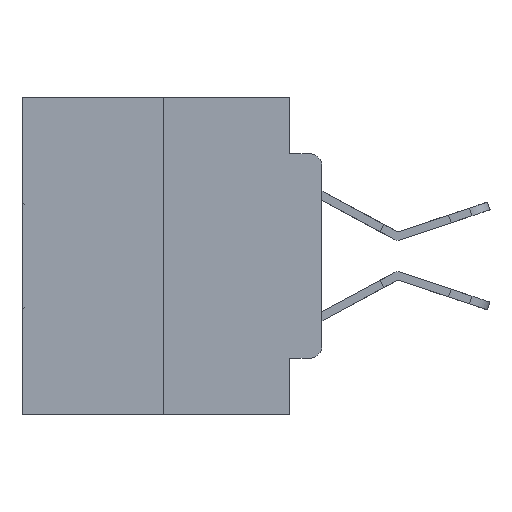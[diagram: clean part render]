
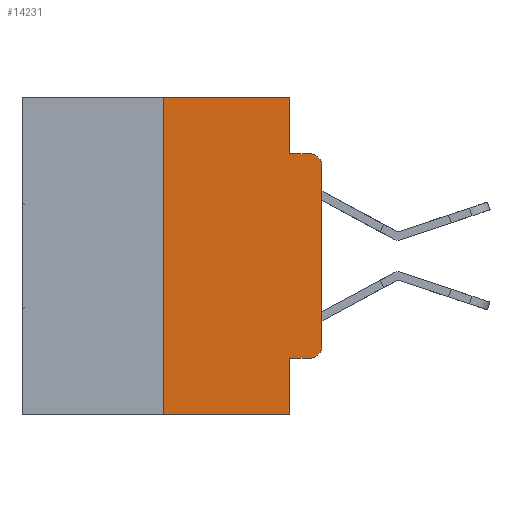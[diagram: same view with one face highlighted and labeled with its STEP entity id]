
A CAD part, left-side view. The second image highlights one B-rep face of the part: STEP entity #14231.
In plain terms, the highlighted planar face has unit normal (-1, 0, 0).
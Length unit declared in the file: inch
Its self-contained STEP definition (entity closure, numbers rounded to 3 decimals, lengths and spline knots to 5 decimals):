
#602 = DIRECTION ( 'NONE',  ( 0., 0., -1. ) ) ;
#644 = CIRCLE ( 'NONE', #16068, 0.02 ) ;
#1045 = ORIENTED_EDGE ( 'NONE', *, *, #2347, .T. ) ;
#1165 = DIRECTION ( 'NONE',  ( 0., -1., 0. ) ) ;
#1322 = LINE ( 'NONE', #6873, #21077 ) ;
#1417 = CARTESIAN_POINT ( 'NONE',  ( 0., 0.051, -0.4115 ) ) ;
#1488 = CARTESIAN_POINT ( 'NONE',  ( 0., 0.051, 0. ) ) ;
#1620 = AXIS2_PLACEMENT_3D ( 'NONE', #18826, #17984, #8869 ) ;
#1840 = ORIENTED_EDGE ( 'NONE', *, *, #3975, .T. ) ;
#2347 = EDGE_CURVE ( 'NONE', #13005, #9622, #16410, .T. ) ;
#3975 = EDGE_CURVE ( 'NONE', #9622, #28104, #10432, .T. ) ;
#4064 = CARTESIAN_POINT ( 'NONE',  ( 0., 0.051, 0. ) ) ;
#4932 = ORIENTED_EDGE ( 'NONE', *, *, #17667, .T. ) ;
#5206 = DIRECTION ( 'NONE',  ( -1., 0., 0. ) ) ;
#6873 = CARTESIAN_POINT ( 'NONE',  ( 0., 0.051, 0. ) ) ;
#6975 = LINE ( 'NONE', #17908, #12547 ) ;
#7841 = LINE ( 'NONE', #13707, #18905 ) ;
#8822 = DIRECTION ( 'NONE',  ( 0., -1., 0. ) ) ;
#8869 = DIRECTION ( 'NONE',  ( 0., 0., -1. ) ) ;
#8878 = VECTOR ( 'NONE', #10041, 39.37008 ) ;
#8889 = EDGE_CURVE ( 'NONE', #18876, #28104, #6975, .T. ) ;
#9395 = LINE ( 'NONE', #11172, #26503 ) ;
#9622 = VERTEX_POINT ( 'NONE', #24877 ) ;
#10041 = DIRECTION ( 'NONE',  ( 0., 0., 1. ) ) ;
#10432 = CIRCLE ( 'NONE', #1620, 0.02 ) ;
#10668 = FACE_OUTER_BOUND ( 'NONE', #19658, .T. ) ;
#10706 = CARTESIAN_POINT ( 'NONE',  ( 0., 0.02, -0.0885 ) ) ;
#11172 = CARTESIAN_POINT ( 'NONE',  ( 0., 0.473, 0. ) ) ;
#11630 = VECTOR ( 'NONE', #15860, 39.37008 ) ;
#12049 = EDGE_CURVE ( 'NONE', #20952, #18876, #24044, .T. ) ;
#12547 = VECTOR ( 'NONE', #1165, 39.37008 ) ;
#12654 = CARTESIAN_POINT ( 'NONE',  ( 0., 0.473, 0. ) ) ;
#12850 = VERTEX_POINT ( 'NONE', #16640 ) ;
#13005 = VERTEX_POINT ( 'NONE', #17226 ) ;
#13604 = EDGE_CURVE ( 'NONE', #12850, #25462, #26732, .T. ) ;
#13707 = CARTESIAN_POINT ( 'NONE',  ( 0., 0.473, -0.5 ) ) ;
#14231 = ADVANCED_FACE ( 'NONE', ( #10668 ), #28911, .F. ) ;
#15016 = DIRECTION ( 'NONE',  ( 1., 0., 0. ) ) ;
#15388 = CARTESIAN_POINT ( 'NONE',  ( 0., 0.051, -0.4115 ) ) ;
#15860 = DIRECTION ( 'NONE',  ( 0., 0., -1. ) ) ;
#16068 = AXIS2_PLACEMENT_3D ( 'NONE', #19388, #5206, #21702 ) ;
#16279 = CARTESIAN_POINT ( 'NONE',  ( 0., 0.051, -0.0885 ) ) ;
#16410 = LINE ( 'NONE', #19671, #28001 ) ;
#16640 = CARTESIAN_POINT ( 'NONE',  ( 0., 0.25, -0.5 ) ) ;
#17096 = CARTESIAN_POINT ( 'NONE',  ( 0., 0.25, 0. ) ) ;
#17226 = CARTESIAN_POINT ( 'NONE',  ( 0., 0., -0.3915 ) ) ;
#17529 = ORIENTED_EDGE ( 'NONE', *, *, #18315, .F. ) ;
#17667 = EDGE_CURVE ( 'NONE', #12850, #22974, #7841, .T. ) ;
#17733 = DIRECTION ( 'NONE',  ( 0., -1., 0. ) ) ;
#17754 = VECTOR ( 'NONE', #17733, 39.37008 ) ;
#17908 = CARTESIAN_POINT ( 'NONE',  ( 0., 0.051, -0.0885 ) ) ;
#17984 = DIRECTION ( 'NONE',  ( -1., 0., 0. ) ) ;
#18315 = EDGE_CURVE ( 'NONE', #24324, #22974, #1322, .T. ) ;
#18519 = LINE ( 'NONE', #15388, #17754 ) ;
#18826 = CARTESIAN_POINT ( 'NONE',  ( 0., 0.02, -0.1085 ) ) ;
#18876 = VERTEX_POINT ( 'NONE', #16279 ) ;
#18905 = VECTOR ( 'NONE', #29908, 39.37008 ) ;
#19388 = CARTESIAN_POINT ( 'NONE',  ( 0., 0.02, -0.3915 ) ) ;
#19631 = DIRECTION ( 'NONE',  ( 0., 0., 1. ) ) ;
#19658 = EDGE_LOOP ( 'NONE', ( #1045, #1840, #20814, #27679, #22287, #28403, #4932, #17529, #30529, #25166 ) ) ;
#19671 = CARTESIAN_POINT ( 'NONE',  ( 0., 0., 0. ) ) ;
#19896 = EDGE_CURVE ( 'NONE', #24324, #21409, #18519, .T. ) ;
#20814 = ORIENTED_EDGE ( 'NONE', *, *, #8889, .F. ) ;
#20952 = VERTEX_POINT ( 'NONE', #4064 ) ;
#21077 = VECTOR ( 'NONE', #23344, 39.37008 ) ;
#21409 = VERTEX_POINT ( 'NONE', #29280 ) ;
#21702 = DIRECTION ( 'NONE',  ( 0., 0., -1. ) ) ;
#22287 = ORIENTED_EDGE ( 'NONE', *, *, #28888, .F. ) ;
#22974 = VERTEX_POINT ( 'NONE', #26177 ) ;
#23344 = DIRECTION ( 'NONE',  ( 0., 0., -1. ) ) ;
#23890 = AXIS2_PLACEMENT_3D ( 'NONE', #12654, #15016, #602 ) ;
#24044 = LINE ( 'NONE', #1488, #11630 ) ;
#24324 = VERTEX_POINT ( 'NONE', #1417 ) ;
#24542 = EDGE_CURVE ( 'NONE', #21409, #13005, #644, .T. ) ;
#24877 = CARTESIAN_POINT ( 'NONE',  ( 0., 0., -0.1085 ) ) ;
#24991 = CARTESIAN_POINT ( 'NONE',  ( 0., 0.25, 0. ) ) ;
#25166 = ORIENTED_EDGE ( 'NONE', *, *, #24542, .T. ) ;
#25462 = VERTEX_POINT ( 'NONE', #24991 ) ;
#26177 = CARTESIAN_POINT ( 'NONE',  ( 0., 0.051, -0.5 ) ) ;
#26503 = VECTOR ( 'NONE', #8822, 39.37008 ) ;
#26732 = LINE ( 'NONE', #17096, #8878 ) ;
#27679 = ORIENTED_EDGE ( 'NONE', *, *, #12049, .F. ) ;
#28001 = VECTOR ( 'NONE', #19631, 39.37008 ) ;
#28104 = VERTEX_POINT ( 'NONE', #10706 ) ;
#28403 = ORIENTED_EDGE ( 'NONE', *, *, #13604, .F. ) ;
#28888 = EDGE_CURVE ( 'NONE', #25462, #20952, #9395, .T. ) ;
#28911 = PLANE ( 'NONE',  #23890 ) ;
#29280 = CARTESIAN_POINT ( 'NONE',  ( 0., 0.02, -0.4115 ) ) ;
#29908 = DIRECTION ( 'NONE',  ( 0., -1., 0. ) ) ;
#30529 = ORIENTED_EDGE ( 'NONE', *, *, #19896, .T. ) ;
